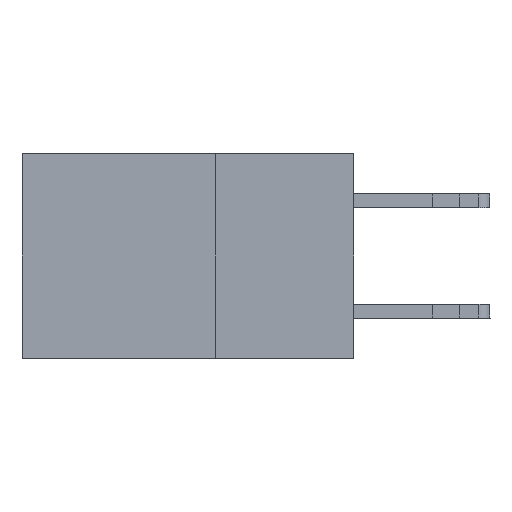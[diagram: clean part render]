
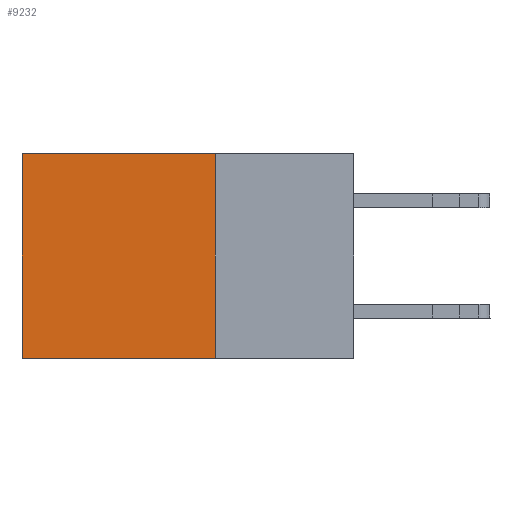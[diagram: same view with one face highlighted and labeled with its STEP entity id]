
A CAD part, left-side view. The second image highlights one B-rep face of the part: STEP entity #9232.
In plain terms, the highlighted planar face has unit normal (-1, 0, 0).
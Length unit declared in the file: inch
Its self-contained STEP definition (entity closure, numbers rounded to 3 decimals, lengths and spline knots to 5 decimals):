
#421 = DIRECTION ( 'NONE',  ( 0., 0., -1. ) ) ;
#1156 = CARTESIAN_POINT ( 'NONE',  ( 0.2875, 0.6, 0. ) ) ;
#1897 = CARTESIAN_POINT ( 'NONE',  ( 0.2875, 0.6, -0.37 ) ) ;
#2353 = EDGE_CURVE ( 'NONE', #20706, #18258, #26328, .T. ) ;
#3120 = DIRECTION ( 'NONE',  ( 0., 1., 0. ) ) ;
#4281 = FACE_OUTER_BOUND ( 'NONE', #5698, .T. ) ;
#5359 = EDGE_CURVE ( 'NONE', #21595, #26143, #11578, .T. ) ;
#5698 = EDGE_LOOP ( 'NONE', ( #11912, #10558, #12914, #13745 ) ) ;
#7620 = CARTESIAN_POINT ( 'NONE',  ( 0.2875, 0.25, 0. ) ) ;
#7659 = EDGE_CURVE ( 'NONE', #18258, #26143, #20247, .T. ) ;
#8296 = CARTESIAN_POINT ( 'NONE',  ( 0.2875, 0.25, 0. ) ) ;
#8983 = CARTESIAN_POINT ( 'NONE',  ( 0.2875, 0.25, -0.37 ) ) ;
#9232 = ADVANCED_FACE ( 'NONE', ( #4281 ), #24691, .F. ) ;
#10292 = DIRECTION ( 'NONE',  ( 0., 0., -1. ) ) ;
#10558 = ORIENTED_EDGE ( 'NONE', *, *, #5359, .F. ) ;
#10960 = CARTESIAN_POINT ( 'NONE',  ( 0.2875, 0.25, -0.37 ) ) ;
#11578 = LINE ( 'NONE', #8983, #14156 ) ;
#11912 = ORIENTED_EDGE ( 'NONE', *, *, #7659, .T. ) ;
#12872 = CARTESIAN_POINT ( 'NONE',  ( 0.2875, 0.25, 0. ) ) ;
#12914 = ORIENTED_EDGE ( 'NONE', *, *, #18837, .F. ) ;
#13745 = ORIENTED_EDGE ( 'NONE', *, *, #2353, .T. ) ;
#14156 = VECTOR ( 'NONE', #3120, 39.37008 ) ;
#14257 = VECTOR ( 'NONE', #21546, 39.37008 ) ;
#17590 = LINE ( 'NONE', #12872, #21367 ) ;
#18238 = DIRECTION ( 'NONE',  ( 0., 1., 0. ) ) ;
#18258 = VERTEX_POINT ( 'NONE', #1156 ) ;
#18837 = EDGE_CURVE ( 'NONE', #20706, #21595, #17590, .T. ) ;
#19520 = CARTESIAN_POINT ( 'NONE',  ( 0.2875, 0.6, 0. ) ) ;
#19562 = AXIS2_PLACEMENT_3D ( 'NONE', #8296, #22476, #10292 ) ;
#20247 = LINE ( 'NONE', #19520, #14257 ) ;
#20706 = VERTEX_POINT ( 'NONE', #7620 ) ;
#20883 = VECTOR ( 'NONE', #18238, 39.37008 ) ;
#21367 = VECTOR ( 'NONE', #421, 39.37008 ) ;
#21546 = DIRECTION ( 'NONE',  ( 0., 0., -1. ) ) ;
#21595 = VERTEX_POINT ( 'NONE', #10960 ) ;
#22476 = DIRECTION ( 'NONE',  ( 1., 0., 0. ) ) ;
#24691 = PLANE ( 'NONE',  #19562 ) ;
#26143 = VERTEX_POINT ( 'NONE', #1897 ) ;
#26168 = CARTESIAN_POINT ( 'NONE',  ( 0.2875, 0.25, 0. ) ) ;
#26328 = LINE ( 'NONE', #26168, #20883 ) ;
